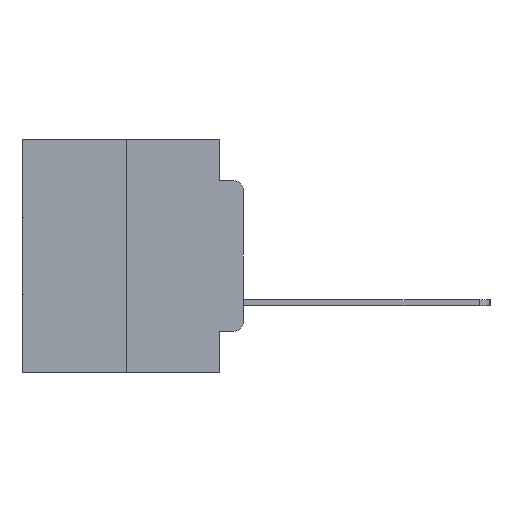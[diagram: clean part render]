
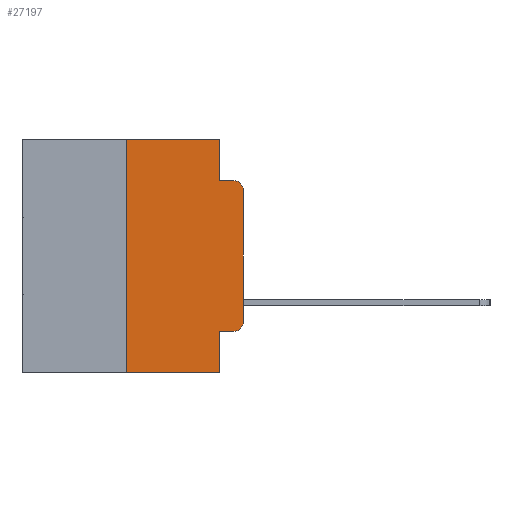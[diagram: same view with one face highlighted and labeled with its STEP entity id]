
A CAD part, left-side view. The second image highlights one B-rep face of the part: STEP entity #27197.
In plain terms, the highlighted planar face has unit normal (-1, 0, 0).
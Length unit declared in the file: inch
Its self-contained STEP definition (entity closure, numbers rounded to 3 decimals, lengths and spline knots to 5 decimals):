
#265 = ORIENTED_EDGE ( 'NONE', *, *, #7726, .F. ) ;
#854 = DIRECTION ( 'NONE',  ( 0., 0., -1. ) ) ;
#957 = ORIENTED_EDGE ( 'NONE', *, *, #18572, .T. ) ;
#1180 = DIRECTION ( 'NONE',  ( 0., 0., -1. ) ) ;
#1619 = VERTEX_POINT ( 'NONE', #25949 ) ;
#1756 = VERTEX_POINT ( 'NONE', #26278 ) ;
#1782 = VECTOR ( 'NONE', #18319, 39.37008 ) ;
#1798 = VERTEX_POINT ( 'NONE', #12638 ) ;
#1823 = CARTESIAN_POINT ( 'NONE',  ( 0., 0.051, -0.0885 ) ) ;
#1835 = ORIENTED_EDGE ( 'NONE', *, *, #4717, .F. ) ;
#2224 = LINE ( 'NONE', #6959, #13399 ) ;
#2553 = VERTEX_POINT ( 'NONE', #4859 ) ;
#2784 = CARTESIAN_POINT ( 'NONE',  ( 0., 0.02, -0.1085 ) ) ;
#3044 = PLANE ( 'NONE',  #12318 ) ;
#3297 = ORIENTED_EDGE ( 'NONE', *, *, #6234, .F. ) ;
#3911 = VERTEX_POINT ( 'NONE', #25051 ) ;
#4717 = EDGE_CURVE ( 'NONE', #12857, #20643, #2224, .T. ) ;
#4859 = CARTESIAN_POINT ( 'NONE',  ( 0., 0.02, -0.0885 ) ) ;
#5076 = DIRECTION ( 'NONE',  ( 0., 0., -1. ) ) ;
#5555 = ORIENTED_EDGE ( 'NONE', *, *, #27366, .F. ) ;
#6150 = LINE ( 'NONE', #1823, #12006 ) ;
#6234 = EDGE_CURVE ( 'NONE', #1619, #6276, #19463, .T. ) ;
#6276 = VERTEX_POINT ( 'NONE', #11794 ) ;
#6959 = CARTESIAN_POINT ( 'NONE',  ( 0., 0.25, 0. ) ) ;
#7165 = AXIS2_PLACEMENT_3D ( 'NONE', #27424, #14516, #1180 ) ;
#7726 = EDGE_CURVE ( 'NONE', #6276, #2553, #6150, .T. ) ;
#8624 = DIRECTION ( 'NONE',  ( 0., -1., 0. ) ) ;
#10212 = DIRECTION ( 'NONE',  ( 0., 0., 1. ) ) ;
#11794 = CARTESIAN_POINT ( 'NONE',  ( 0., 0.051, -0.0885 ) ) ;
#11966 = ORIENTED_EDGE ( 'NONE', *, *, #12533, .T. ) ;
#12006 = VECTOR ( 'NONE', #16208, 39.37008 ) ;
#12256 = CARTESIAN_POINT ( 'NONE',  ( 0., 0.051, 0. ) ) ;
#12318 = AXIS2_PLACEMENT_3D ( 'NONE', #27119, #14209, #854 ) ;
#12533 = EDGE_CURVE ( 'NONE', #12857, #13792, #28226, .T. ) ;
#12591 = VECTOR ( 'NONE', #19284, 39.37008 ) ;
#12638 = CARTESIAN_POINT ( 'NONE',  ( 0., 0.02, -0.4115 ) ) ;
#12857 = VERTEX_POINT ( 'NONE', #22818 ) ;
#13399 = VECTOR ( 'NONE', #22173, 39.37008 ) ;
#13538 = DIRECTION ( 'NONE',  ( 0., -1., 0. ) ) ;
#13792 = VERTEX_POINT ( 'NONE', #23910 ) ;
#14209 = DIRECTION ( 'NONE',  ( 1., 0., 0. ) ) ;
#14516 = DIRECTION ( 'NONE',  ( -1., 0., 0. ) ) ;
#14530 = LINE ( 'NONE', #21071, #19680 ) ;
#15077 = EDGE_CURVE ( 'NONE', #3911, #2553, #23017, .T. ) ;
#15831 = VECTOR ( 'NONE', #13538, 39.37008 ) ;
#16208 = DIRECTION ( 'NONE',  ( 0., -1., 0. ) ) ;
#16555 = EDGE_CURVE ( 'NONE', #18819, #3911, #23658, .T. ) ;
#16666 = ORIENTED_EDGE ( 'NONE', *, *, #16555, .T. ) ;
#16685 = AXIS2_PLACEMENT_3D ( 'NONE', #2784, #18277, #5076 ) ;
#16765 = CARTESIAN_POINT ( 'NONE',  ( 0., 0., 0. ) ) ;
#17169 = CARTESIAN_POINT ( 'NONE',  ( 0., 0.051, 0. ) ) ;
#17737 = LINE ( 'NONE', #17169, #12591 ) ;
#17896 = VECTOR ( 'NONE', #10212, 39.37008 ) ;
#18037 = EDGE_LOOP ( 'NONE', ( #16666, #19664, #265, #3297, #5555, #1835, #11966, #20960, #25018, #957 ) ) ;
#18277 = DIRECTION ( 'NONE',  ( -1., 0., 0. ) ) ;
#18319 = DIRECTION ( 'NONE',  ( 0., 0., -1. ) ) ;
#18572 = EDGE_CURVE ( 'NONE', #1798, #18819, #21838, .T. ) ;
#18669 = FACE_OUTER_BOUND ( 'NONE', #18037, .T. ) ;
#18819 = VERTEX_POINT ( 'NONE', #21840 ) ;
#19109 = DIRECTION ( 'NONE',  ( 0., -1., 0. ) ) ;
#19284 = DIRECTION ( 'NONE',  ( 0., 0., -1. ) ) ;
#19461 = CARTESIAN_POINT ( 'NONE',  ( 0., 0.473, -0.5 ) ) ;
#19463 = LINE ( 'NONE', #12256, #1782 ) ;
#19664 = ORIENTED_EDGE ( 'NONE', *, *, #15077, .T. ) ;
#19680 = VECTOR ( 'NONE', #19109, 39.37008 ) ;
#20568 = VECTOR ( 'NONE', #8624, 39.37008 ) ;
#20643 = VERTEX_POINT ( 'NONE', #21181 ) ;
#20960 = ORIENTED_EDGE ( 'NONE', *, *, #25766, .F. ) ;
#21071 = CARTESIAN_POINT ( 'NONE',  ( 0., 0.473, 0. ) ) ;
#21181 = CARTESIAN_POINT ( 'NONE',  ( 0., 0.25, 0. ) ) ;
#21464 = EDGE_CURVE ( 'NONE', #1756, #1798, #27254, .T. ) ;
#21838 = CIRCLE ( 'NONE', #7165, 0.02 ) ;
#21840 = CARTESIAN_POINT ( 'NONE',  ( 0., 0., -0.3915 ) ) ;
#22173 = DIRECTION ( 'NONE',  ( 0., 0., 1. ) ) ;
#22818 = CARTESIAN_POINT ( 'NONE',  ( 0., 0.25, -0.5 ) ) ;
#23017 = CIRCLE ( 'NONE', #16685, 0.02 ) ;
#23658 = LINE ( 'NONE', #16765, #17896 ) ;
#23910 = CARTESIAN_POINT ( 'NONE',  ( 0., 0.051, -0.5 ) ) ;
#25018 = ORIENTED_EDGE ( 'NONE', *, *, #21464, .T. ) ;
#25051 = CARTESIAN_POINT ( 'NONE',  ( 0., 0., -0.1085 ) ) ;
#25766 = EDGE_CURVE ( 'NONE', #1756, #13792, #17737, .T. ) ;
#25949 = CARTESIAN_POINT ( 'NONE',  ( 0., 0.051, 0. ) ) ;
#26278 = CARTESIAN_POINT ( 'NONE',  ( 0., 0.051, -0.4115 ) ) ;
#26459 = CARTESIAN_POINT ( 'NONE',  ( 0., 0.051, -0.4115 ) ) ;
#27119 = CARTESIAN_POINT ( 'NONE',  ( 0., 0.473, 0. ) ) ;
#27197 = ADVANCED_FACE ( 'NONE', ( #18669 ), #3044, .F. ) ;
#27254 = LINE ( 'NONE', #26459, #15831 ) ;
#27366 = EDGE_CURVE ( 'NONE', #20643, #1619, #14530, .T. ) ;
#27424 = CARTESIAN_POINT ( 'NONE',  ( 0., 0.02, -0.3915 ) ) ;
#28226 = LINE ( 'NONE', #19461, #20568 ) ;
